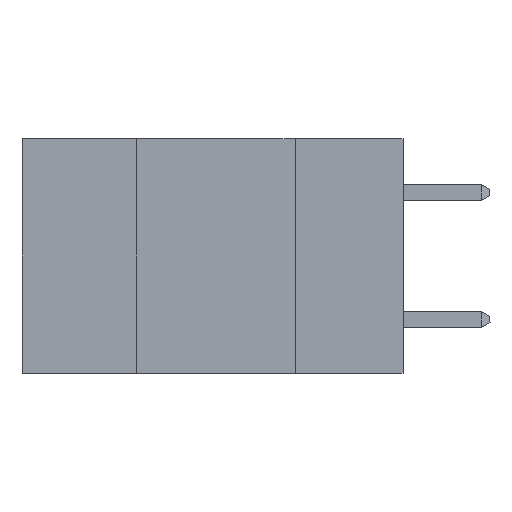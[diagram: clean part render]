
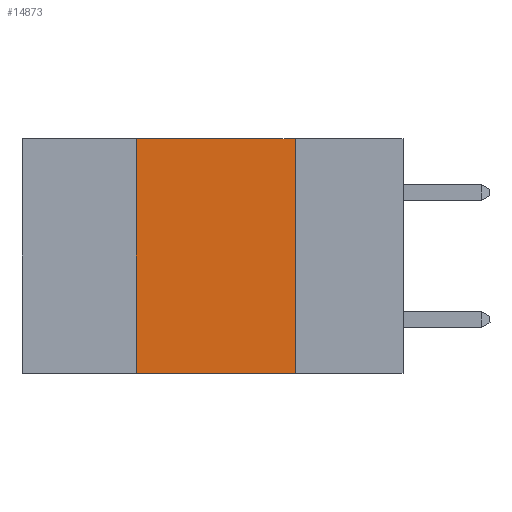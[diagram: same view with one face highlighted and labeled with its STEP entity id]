
A CAD part, left-side view. The second image highlights one B-rep face of the part: STEP entity #14873.
In plain terms, the highlighted planar face has unit normal (-1, 0, 0).
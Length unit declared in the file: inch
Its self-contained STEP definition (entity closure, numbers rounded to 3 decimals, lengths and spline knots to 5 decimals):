
#226 = EDGE_CURVE ( 'NONE', #1190, #1787, #19205, .T. ) ;
#1190 = VERTEX_POINT ( 'NONE', #4334 ) ;
#1787 = VERTEX_POINT ( 'NONE', #10394 ) ;
#1836 = DIRECTION ( 'NONE',  ( 0., -1., 0. ) ) ;
#2098 = DIRECTION ( 'NONE',  ( 0., -1., 0. ) ) ;
#3449 = VECTOR ( 'NONE', #1836, 39.37008 ) ;
#3589 = CARTESIAN_POINT ( 'NONE',  ( 0., 0.17, 0. ) ) ;
#3805 = LINE ( 'NONE', #3589, #7427 ) ;
#3934 = LINE ( 'NONE', #5013, #3449 ) ;
#4028 = ORIENTED_EDGE ( 'NONE', *, *, #10855, .F. ) ;
#4334 = CARTESIAN_POINT ( 'NONE',  ( 0., 0.42, -0.37 ) ) ;
#4411 = PLANE ( 'NONE',  #19727 ) ;
#5013 = CARTESIAN_POINT ( 'NONE',  ( 0., 0.6, 0. ) ) ;
#5822 = FACE_OUTER_BOUND ( 'NONE', #13066, .T. ) ;
#6609 = CARTESIAN_POINT ( 'NONE',  ( 0., 0.17, 0. ) ) ;
#6742 = CARTESIAN_POINT ( 'NONE',  ( 0., 0.6, -0.37 ) ) ;
#7427 = VECTOR ( 'NONE', #16013, 39.37008 ) ;
#7619 = VECTOR ( 'NONE', #2098, 39.37008 ) ;
#9039 = CARTESIAN_POINT ( 'NONE',  ( 0., 0.6, 0. ) ) ;
#9556 = ORIENTED_EDGE ( 'NONE', *, *, #14420, .F. ) ;
#10052 = VECTOR ( 'NONE', #16689, 39.37008 ) ;
#10394 = CARTESIAN_POINT ( 'NONE',  ( 0., 0.42, 0. ) ) ;
#10637 = DIRECTION ( 'NONE',  ( 0., 0., -1. ) ) ;
#10855 = EDGE_CURVE ( 'NONE', #17830, #18289, #3805, .T. ) ;
#13066 = EDGE_LOOP ( 'NONE', ( #4028, #9556, #19612, #13197 ) ) ;
#13197 = ORIENTED_EDGE ( 'NONE', *, *, #17910, .T. ) ;
#14420 = EDGE_CURVE ( 'NONE', #1787, #17830, #3934, .T. ) ;
#14873 = ADVANCED_FACE ( 'NONE', ( #5822 ), #4411, .F. ) ;
#16013 = DIRECTION ( 'NONE',  ( 0., 0., -1. ) ) ;
#16689 = DIRECTION ( 'NONE',  ( 0., 0., 1. ) ) ;
#17651 = CARTESIAN_POINT ( 'NONE',  ( 0., 0.17, -0.37 ) ) ;
#17830 = VERTEX_POINT ( 'NONE', #6609 ) ;
#17910 = EDGE_CURVE ( 'NONE', #1190, #18289, #19431, .T. ) ;
#18289 = VERTEX_POINT ( 'NONE', #17651 ) ;
#19205 = LINE ( 'NONE', #19209, #10052 ) ;
#19209 = CARTESIAN_POINT ( 'NONE',  ( 0., 0.42, 0. ) ) ;
#19431 = LINE ( 'NONE', #6742, #7619 ) ;
#19612 = ORIENTED_EDGE ( 'NONE', *, *, #226, .F. ) ;
#19727 = AXIS2_PLACEMENT_3D ( 'NONE', #9039, #19828, #10637 ) ;
#19828 = DIRECTION ( 'NONE',  ( 1., 0., 0. ) ) ;
